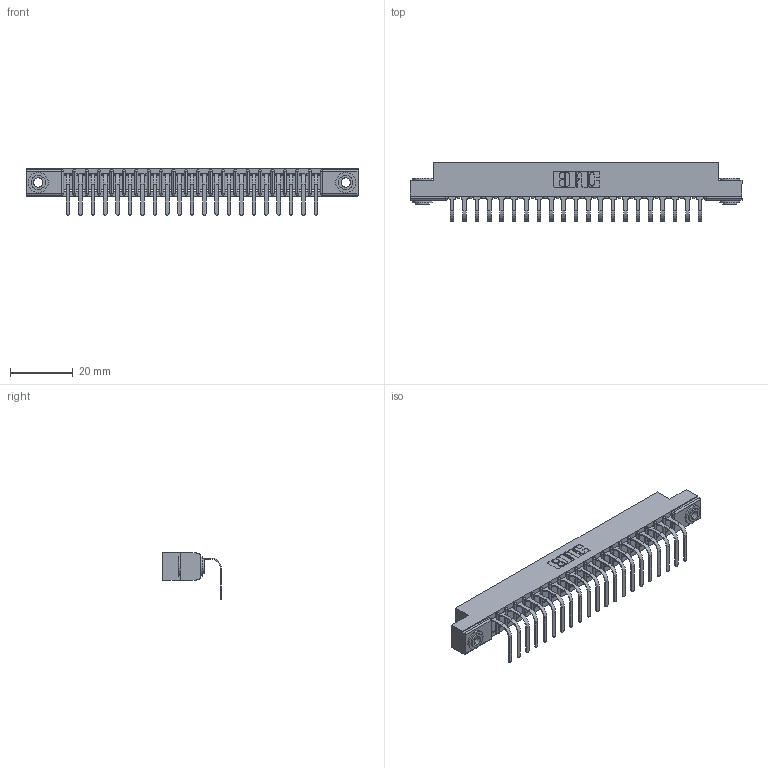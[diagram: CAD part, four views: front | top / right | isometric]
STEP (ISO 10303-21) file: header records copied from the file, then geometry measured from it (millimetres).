
FILE_DESCRIPTION (( 'STEP AP203' ), '1' );
FILE_NAME ('357-021-558-103.STEP', '2022-07-13T21:00:05', ( '' ), ( '' ), 'SwSTEP 2.0', 'SolidWorks 2020', '' );
FILE_SCHEMA (( 'CONFIG_CONTROL_DESIGN' ));
Length unit declared in the file: inch
Products named in the file (4): 357-021-558-103; 307 Part_.156 Dia Mounting Holes; 345-250-002_345-250-002-102; 307-290-001_558 - 2 (Single)
Assembly tree (24 placements, depth 2):
  357-021-558-103
    307 Part_.156 Dia Mounting Holes
    307-290-001_558 - 2 (Single)  x21
    345-250-002_345-250-002-102  x2
Bounding box: 106.22 x 18.78 x 14.81 mm (x, y, z)
Volume: 6796.8 mm3; surface area: 11274.7 mm2
Topology: 24 solids, 24 shells, 1452 faces, 4089 edges, 2634 vertices
Faces by surface type: plane 913, cylinder 487, sphere 44, cone 8
Entity records: 21761 total; most frequent: CARTESIAN_POINT 3637, ORIENTED_EDGE 3614, DIRECTION 3565, EDGE_CURVE 1807, LINE 1369, VECTOR 1369, VERTEX_POINT 1170, AXIS2_PLACEMENT_3D 1098
